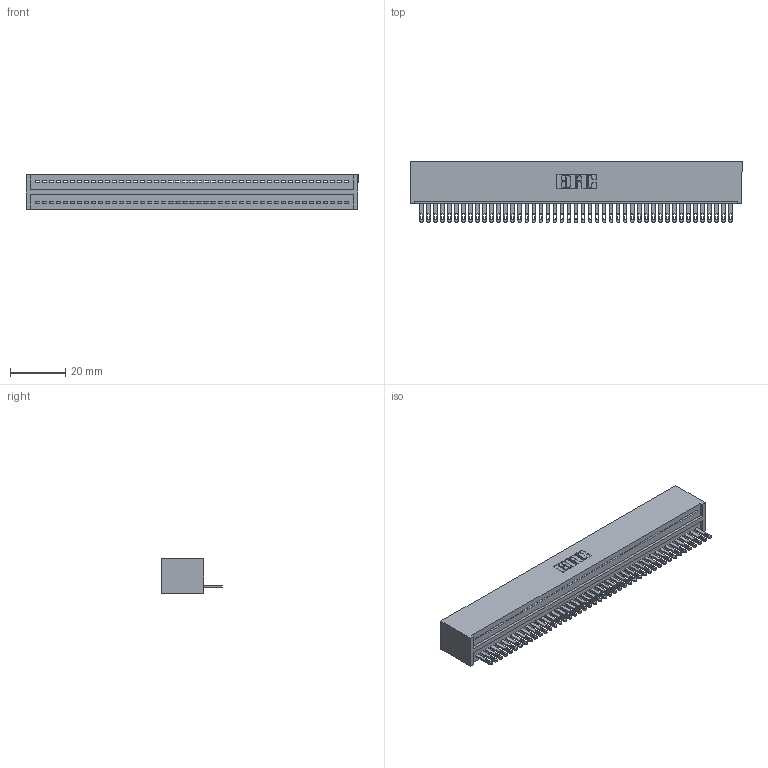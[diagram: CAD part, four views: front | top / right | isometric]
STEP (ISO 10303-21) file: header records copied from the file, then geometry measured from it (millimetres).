
FILE_DESCRIPTION (( 'STEP AP203' ), '1' );
FILE_NAME ('325-045-500-101.STEP', '2020-02-24T22:34:36', ( '' ), ( '' ), 'SwSTEP 2.0', 'SolidWorks 2016', '' );
FILE_SCHEMA (( 'CONFIG_CONTROL_DESIGN' ));
Length unit declared in the file: inch
Products named in the file (3): 325-292-001_325-293-100; 325 Part_Lugless; 325-045-500-101
Assembly tree (46 placements, depth 2):
  325-045-500-101
    325 Part_Lugless
    325-292-001_325-293-100  x45
Bounding box: 119.94 x 21.84 x 12.45 mm (x, y, z)
Volume: 15849.5 mm3; surface area: 17962.1 mm2
Topology: 46 solids, 46 shells, 2536 faces, 7847 edges, 5230 vertices
Faces by surface type: plane 1686, cylinder 850
Entity records: 26775 total; most frequent: CARTESIAN_POINT 4625, ORIENTED_EDGE 4606, DIRECTION 3889, EDGE_CURVE 2303, VECTOR 2179, LINE 2179, VERTEX_POINT 1534, AXIS2_PLACEMENT_3D 855
